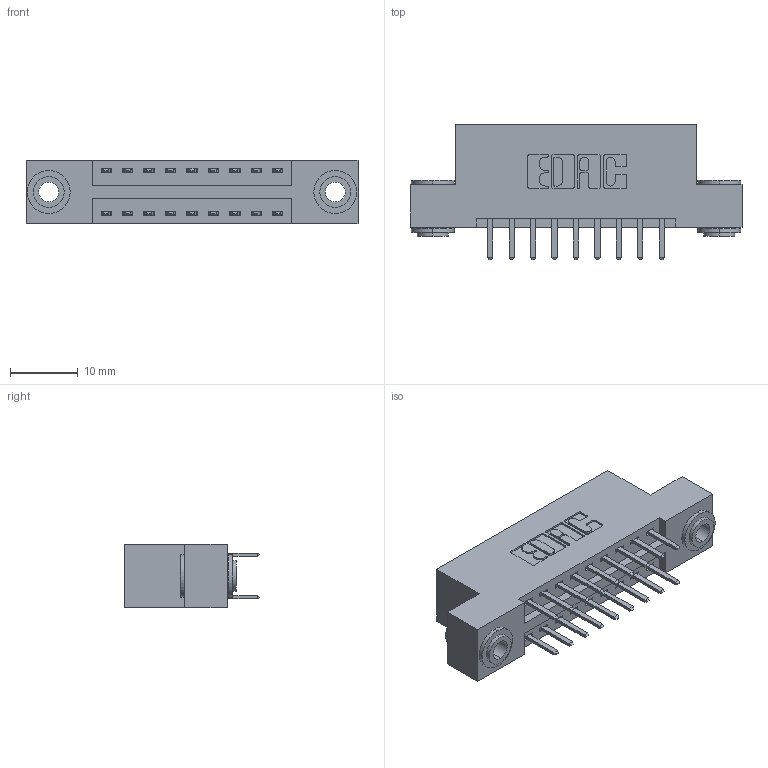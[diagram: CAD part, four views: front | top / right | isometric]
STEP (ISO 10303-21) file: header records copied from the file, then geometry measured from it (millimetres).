
FILE_DESCRIPTION (( 'STEP AP203' ), '1' );
FILE_NAME ('396-018-520-203.STEP', '2019-10-30T02:45:14', ( '' ), ( '' ), 'SwSTEP 2.0', 'SolidWorks 2016', '' );
FILE_SCHEMA (( 'CONFIG_CONTROL_DESIGN' ));
Length unit declared in the file: inch
Products named in the file (4): 396-018-520-203; 346 Part_Flush Mounting Lugs - 0.156 Dia-TH; 345-292-001_345-293-120; 345-250-002_345-250-002-102
Assembly tree (21 placements, depth 2):
  396-018-520-203
    346 Part_Flush Mounting Lugs - 0.156 Dia-TH
    345-292-001_345-293-120  x18
    345-250-002_345-250-002-102  x2
Bounding box: 49.15 x 20.02 x 9.4 mm (x, y, z)
Volume: 4547.8 mm3; surface area: 5928.2 mm2
Topology: 21 solids, 21 shells, 1168 faces, 3339 edges, 2174 vertices
Faces by surface type: plane 752, cylinder 408, cone 8
Entity records: 11080 total; most frequent: CARTESIAN_POINT 1859, ORIENTED_EDGE 1774, DIRECTION 1709, EDGE_CURVE 887, VECTOR 691, LINE 691, VERTEX_POINT 586, AXIS2_PLACEMENT_3D 509
